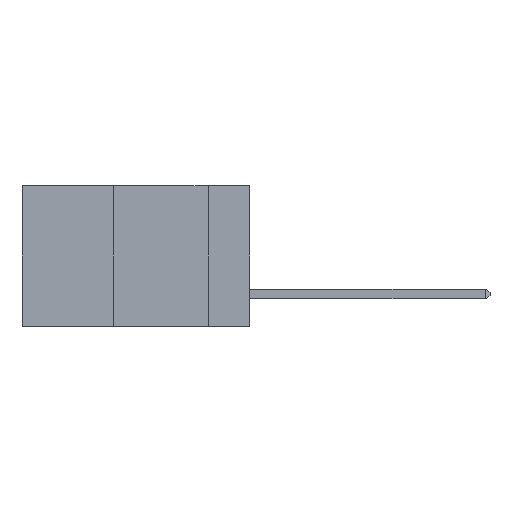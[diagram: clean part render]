
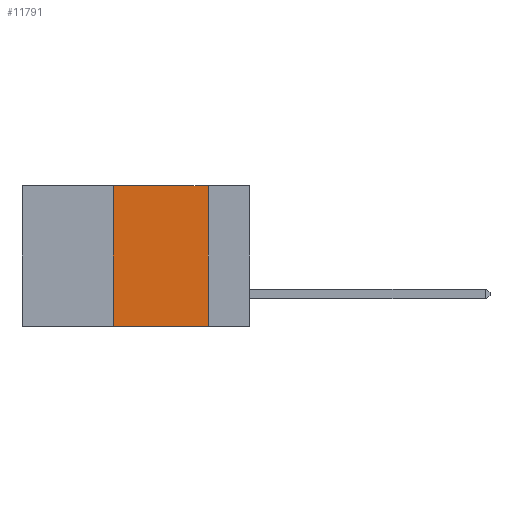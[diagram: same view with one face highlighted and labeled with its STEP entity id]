
A CAD part, left-side view. The second image highlights one B-rep face of the part: STEP entity #11791.
In plain terms, the highlighted planar face has unit normal (-1, 0, 0).
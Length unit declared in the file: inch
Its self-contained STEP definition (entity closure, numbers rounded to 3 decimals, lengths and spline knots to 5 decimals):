
#137 = ORIENTED_EDGE ( 'NONE', *, *, #12543, .T. ) ;
#191 = VERTEX_POINT ( 'NONE', #18797 ) ;
#327 = PLANE ( 'NONE',  #419 ) ;
#419 = AXIS2_PLACEMENT_3D ( 'NONE', #18864, #13005, #3539 ) ;
#436 = DIRECTION ( 'NONE',  ( 0., 0., -1. ) ) ;
#833 = VECTOR ( 'NONE', #436, 39.37008 ) ;
#903 = ORIENTED_EDGE ( 'NONE', *, *, #4759, .F. ) ;
#987 = ORIENTED_EDGE ( 'NONE', *, *, #17500, .F. ) ;
#1333 = ORIENTED_EDGE ( 'NONE', *, *, #14087, .F. ) ;
#1486 = VERTEX_POINT ( 'NONE', #15633 ) ;
#2745 = EDGE_LOOP ( 'NONE', ( #903, #1333, #987, #137 ) ) ;
#3498 = DIRECTION ( 'NONE',  ( 0., 0., 1. ) ) ;
#3539 = DIRECTION ( 'NONE',  ( 0., 0., -1. ) ) ;
#4551 = VECTOR ( 'NONE', #12851, 39.37008 ) ;
#4759 = EDGE_CURVE ( 'NONE', #191, #1486, #5041, .T. ) ;
#5041 = LINE ( 'NONE', #17465, #833 ) ;
#5769 = CARTESIAN_POINT ( 'NONE',  ( 0., 0.36, 0. ) ) ;
#6089 = LINE ( 'NONE', #7659, #13920 ) ;
#7659 = CARTESIAN_POINT ( 'NONE',  ( 0., 0.6, -0.37 ) ) ;
#11279 = CARTESIAN_POINT ( 'NONE',  ( 0., 0.6, 0. ) ) ;
#11791 = ADVANCED_FACE ( 'NONE', ( #19037 ), #327, .F. ) ;
#12543 = EDGE_CURVE ( 'NONE', #16536, #1486, #6089, .T. ) ;
#12851 = DIRECTION ( 'NONE',  ( 0., -1., 0. ) ) ;
#12963 = LINE ( 'NONE', #11279, #4551 ) ;
#12971 = CARTESIAN_POINT ( 'NONE',  ( 0., 0.36, 0. ) ) ;
#13005 = DIRECTION ( 'NONE',  ( 1., 0., 0. ) ) ;
#13920 = VECTOR ( 'NONE', #18297, 39.37008 ) ;
#13943 = CARTESIAN_POINT ( 'NONE',  ( 0., 0.36, -0.37 ) ) ;
#14087 = EDGE_CURVE ( 'NONE', #19846, #191, #12963, .T. ) ;
#15491 = VECTOR ( 'NONE', #3498, 39.37008 ) ;
#15633 = CARTESIAN_POINT ( 'NONE',  ( 0., 0.11, -0.37 ) ) ;
#16536 = VERTEX_POINT ( 'NONE', #13943 ) ;
#17465 = CARTESIAN_POINT ( 'NONE',  ( 0., 0.11, 0. ) ) ;
#17500 = EDGE_CURVE ( 'NONE', #16536, #19846, #19453, .T. ) ;
#18297 = DIRECTION ( 'NONE',  ( 0., -1., 0. ) ) ;
#18797 = CARTESIAN_POINT ( 'NONE',  ( 0., 0.11, 0. ) ) ;
#18864 = CARTESIAN_POINT ( 'NONE',  ( 0., 0.6, 0. ) ) ;
#19037 = FACE_OUTER_BOUND ( 'NONE', #2745, .T. ) ;
#19453 = LINE ( 'NONE', #12971, #15491 ) ;
#19846 = VERTEX_POINT ( 'NONE', #5769 ) ;
